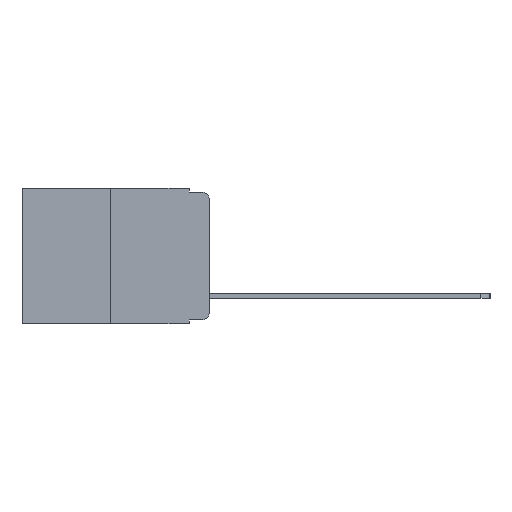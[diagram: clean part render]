
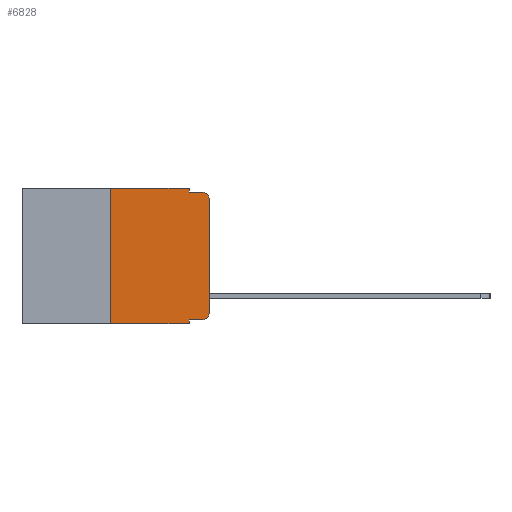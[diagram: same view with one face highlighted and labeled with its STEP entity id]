
A CAD part, left-side view. The second image highlights one B-rep face of the part: STEP entity #6828.
In plain terms, the highlighted planar face has unit normal (-1, 0, 0).
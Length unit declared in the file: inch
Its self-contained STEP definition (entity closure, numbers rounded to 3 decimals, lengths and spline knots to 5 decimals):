
#545 = VERTEX_POINT ( 'NONE', #11022 ) ;
#892 = CARTESIAN_POINT ( 'NONE',  ( 0., 0.051, -0.333 ) ) ;
#988 = DIRECTION ( 'NONE',  ( -1., 0., 0. ) ) ;
#990 = VECTOR ( 'NONE', #7390, 39.37008 ) ;
#1303 = DIRECTION ( 'NONE',  ( 0., 0., -1. ) ) ;
#3144 = ORIENTED_EDGE ( 'NONE', *, *, #7997, .T. ) ;
#3146 = VERTEX_POINT ( 'NONE', #16744 ) ;
#3384 = DIRECTION ( 'NONE',  ( 0., 0., -1. ) ) ;
#3385 = ORIENTED_EDGE ( 'NONE', *, *, #13304, .T. ) ;
#3747 = CARTESIAN_POINT ( 'NONE',  ( 0., 0.051, -0.01 ) ) ;
#3976 = VERTEX_POINT ( 'NONE', #6823 ) ;
#4471 = DIRECTION ( 'NONE',  ( -1., 0., 0. ) ) ;
#4480 = CARTESIAN_POINT ( 'NONE',  ( 0., 0.25, 0. ) ) ;
#5018 = EDGE_CURVE ( 'NONE', #13166, #17623, #14536, .T. ) ;
#5134 = LINE ( 'NONE', #13075, #12012 ) ;
#5168 = EDGE_CURVE ( 'NONE', #8205, #11916, #5134, .T. ) ;
#5314 = ORIENTED_EDGE ( 'NONE', *, *, #5168, .F. ) ;
#6001 = VECTOR ( 'NONE', #15210, 39.37008 ) ;
#6033 = CARTESIAN_POINT ( 'NONE',  ( 0., 0.051, 0. ) ) ;
#6270 = ORIENTED_EDGE ( 'NONE', *, *, #9353, .T. ) ;
#6411 = CARTESIAN_POINT ( 'NONE',  ( 0., 0.051, 0. ) ) ;
#6575 = VERTEX_POINT ( 'NONE', #16057 ) ;
#6823 = CARTESIAN_POINT ( 'NONE',  ( 0., 0.02, -0.01 ) ) ;
#6828 = ADVANCED_FACE ( 'NONE', ( #14885 ), #8739, .F. ) ;
#7390 = DIRECTION ( 'NONE',  ( 0., -1., 0. ) ) ;
#7649 = ORIENTED_EDGE ( 'NONE', *, *, #5018, .T. ) ;
#7838 = CARTESIAN_POINT ( 'NONE',  ( 0., 0.02, -0.333 ) ) ;
#7862 = ORIENTED_EDGE ( 'NONE', *, *, #12376, .T. ) ;
#7997 = EDGE_CURVE ( 'NONE', #15780, #13166, #15643, .T. ) ;
#8205 = VERTEX_POINT ( 'NONE', #4480 ) ;
#8248 = DIRECTION ( 'NONE',  ( 0., -1., 0. ) ) ;
#8646 = LINE ( 'NONE', #3747, #11690 ) ;
#8709 = ORIENTED_EDGE ( 'NONE', *, *, #10612, .F. ) ;
#8739 = PLANE ( 'NONE',  #15174 ) ;
#8900 = EDGE_CURVE ( 'NONE', #15780, #9007, #15866, .T. ) ;
#8927 = AXIS2_PLACEMENT_3D ( 'NONE', #9952, #988, #11228 ) ;
#9007 = VERTEX_POINT ( 'NONE', #10650 ) ;
#9327 = VECTOR ( 'NONE', #3384, 39.37008 ) ;
#9353 = EDGE_CURVE ( 'NONE', #3146, #9007, #17025, .T. ) ;
#9688 = VECTOR ( 'NONE', #1303, 39.37008 ) ;
#9761 = EDGE_CURVE ( 'NONE', #3146, #8205, #17226, .T. ) ;
#9952 = CARTESIAN_POINT ( 'NONE',  ( 0., 0.02, -0.03 ) ) ;
#10045 = DIRECTION ( 'NONE',  ( 0., 0., -1. ) ) ;
#10194 = AXIS2_PLACEMENT_3D ( 'NONE', #12785, #4471, #14111 ) ;
#10484 = CARTESIAN_POINT ( 'NONE',  ( 0., 0.051, 0. ) ) ;
#10612 = EDGE_CURVE ( 'NONE', #11916, #545, #13207, .T. ) ;
#10650 = CARTESIAN_POINT ( 'NONE',  ( 0., 0.051, -0.343 ) ) ;
#11022 = CARTESIAN_POINT ( 'NONE',  ( 0., 0.051, -0.01 ) ) ;
#11228 = DIRECTION ( 'NONE',  ( 0., 0., -1. ) ) ;
#11481 = EDGE_CURVE ( 'NONE', #545, #3976, #8646, .T. ) ;
#11690 = VECTOR ( 'NONE', #8248, 39.37008 ) ;
#11916 = VERTEX_POINT ( 'NONE', #6411 ) ;
#11955 = CARTESIAN_POINT ( 'NONE',  ( 0., 0., 0. ) ) ;
#12012 = VECTOR ( 'NONE', #18174, 39.37008 ) ;
#12376 = EDGE_CURVE ( 'NONE', #6575, #3976, #14073, .T. ) ;
#12629 = CARTESIAN_POINT ( 'NONE',  ( 0., 0.473, 0. ) ) ;
#12785 = CARTESIAN_POINT ( 'NONE',  ( 0., 0.02, -0.313 ) ) ;
#13075 = CARTESIAN_POINT ( 'NONE',  ( 0., 0.473, 0. ) ) ;
#13166 = VERTEX_POINT ( 'NONE', #7838 ) ;
#13207 = LINE ( 'NONE', #6033, #9688 ) ;
#13304 = EDGE_CURVE ( 'NONE', #17623, #6575, #16838, .T. ) ;
#13323 = DIRECTION ( 'NONE',  ( 0., 0., 1. ) ) ;
#13423 = VECTOR ( 'NONE', #13323, 39.37008 ) ;
#13845 = VECTOR ( 'NONE', #15168, 39.37008 ) ;
#13912 = CARTESIAN_POINT ( 'NONE',  ( 0., 0.473, -0.343 ) ) ;
#13979 = EDGE_LOOP ( 'NONE', ( #3385, #7862, #18199, #8709, #5314, #16464, #6270, #17235, #3144, #7649 ) ) ;
#14073 = CIRCLE ( 'NONE', #8927, 0.02 ) ;
#14111 = DIRECTION ( 'NONE',  ( 0., 0., -1. ) ) ;
#14536 = CIRCLE ( 'NONE', #10194, 0.02 ) ;
#14885 = FACE_OUTER_BOUND ( 'NONE', #13979, .T. ) ;
#15168 = DIRECTION ( 'NONE',  ( 0., 0., 1. ) ) ;
#15174 = AXIS2_PLACEMENT_3D ( 'NONE', #12629, #17791, #10045 ) ;
#15210 = DIRECTION ( 'NONE',  ( 0., -1., 0. ) ) ;
#15315 = CARTESIAN_POINT ( 'NONE',  ( 0., 0.051, -0.333 ) ) ;
#15643 = LINE ( 'NONE', #15315, #990 ) ;
#15780 = VERTEX_POINT ( 'NONE', #892 ) ;
#15866 = LINE ( 'NONE', #10484, #9327 ) ;
#16057 = CARTESIAN_POINT ( 'NONE',  ( 0., 0., -0.03 ) ) ;
#16464 = ORIENTED_EDGE ( 'NONE', *, *, #9761, .F. ) ;
#16618 = CARTESIAN_POINT ( 'NONE',  ( 0., 0., -0.313 ) ) ;
#16744 = CARTESIAN_POINT ( 'NONE',  ( 0., 0.25, -0.343 ) ) ;
#16838 = LINE ( 'NONE', #11955, #13423 ) ;
#17025 = LINE ( 'NONE', #13912, #6001 ) ;
#17226 = LINE ( 'NONE', #17696, #13845 ) ;
#17235 = ORIENTED_EDGE ( 'NONE', *, *, #8900, .F. ) ;
#17623 = VERTEX_POINT ( 'NONE', #16618 ) ;
#17696 = CARTESIAN_POINT ( 'NONE',  ( 0., 0.25, 0. ) ) ;
#17791 = DIRECTION ( 'NONE',  ( 1., 0., 0. ) ) ;
#18174 = DIRECTION ( 'NONE',  ( 0., -1., 0. ) ) ;
#18199 = ORIENTED_EDGE ( 'NONE', *, *, #11481, .F. ) ;
